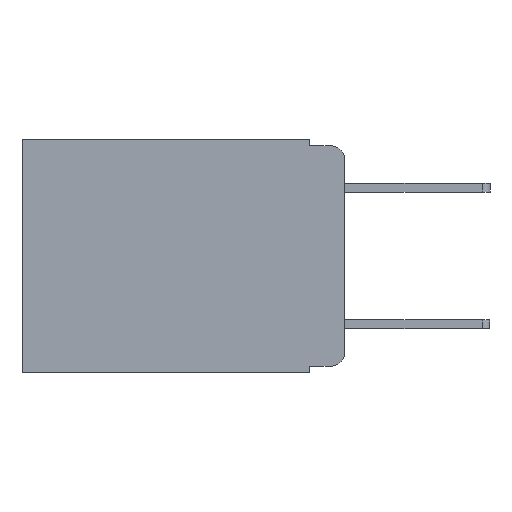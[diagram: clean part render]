
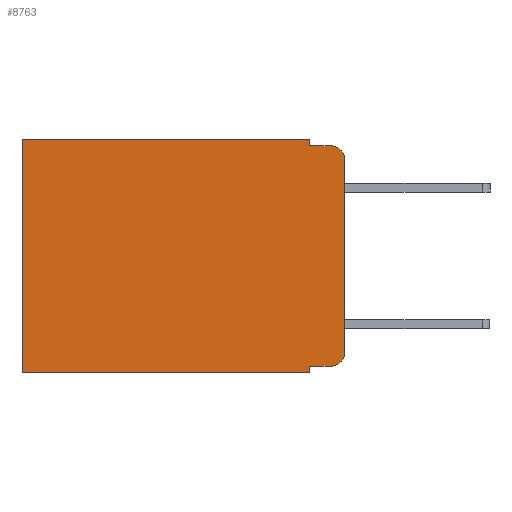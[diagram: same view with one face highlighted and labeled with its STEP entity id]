
A CAD part, left-side view. The second image highlights one B-rep face of the part: STEP entity #8763.
In plain terms, the highlighted planar face has unit normal (-1, 0, 0).
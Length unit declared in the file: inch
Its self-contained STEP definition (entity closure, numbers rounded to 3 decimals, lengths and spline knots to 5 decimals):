
#211 = VERTEX_POINT ( 'NONE', #2208 ) ;
#552 = DIRECTION ( 'NONE',  ( 0., 1., 0. ) ) ;
#572 = AXIS2_PLACEMENT_3D ( 'NONE', #5854, #4421, #10135 ) ;
#586 = CARTESIAN_POINT ( 'NONE',  ( 0.298, 0.051, -0.01 ) ) ;
#805 = VERTEX_POINT ( 'NONE', #586 ) ;
#829 = LINE ( 'NONE', #3305, #9333 ) ;
#880 = EDGE_CURVE ( 'NONE', #4049, #7673, #10518, .T. ) ;
#960 = CARTESIAN_POINT ( 'NONE',  ( 0.298, 0.051, 0. ) ) ;
#988 = EDGE_LOOP ( 'NONE', ( #2764, #4732, #3304, #2114, #5813, #4872, #7595, #1757, #4469, #1127 ) ) ;
#992 = EDGE_CURVE ( 'NONE', #5598, #4135, #9560, .T. ) ;
#1011 = EDGE_CURVE ( 'NONE', #8769, #5960, #829, .T. ) ;
#1127 = ORIENTED_EDGE ( 'NONE', *, *, #2802, .T. ) ;
#1315 = DIRECTION ( 'NONE',  ( 0., 0., -1. ) ) ;
#1406 = AXIS2_PLACEMENT_3D ( 'NONE', #4941, #5528, #5563 ) ;
#1739 = CARTESIAN_POINT ( 'NONE',  ( 0.298, 0.051, -0.343 ) ) ;
#1757 = ORIENTED_EDGE ( 'NONE', *, *, #4881, .F. ) ;
#1836 = VECTOR ( 'NONE', #6112, 39.37008 ) ;
#1850 = LINE ( 'NONE', #960, #3791 ) ;
#2114 = ORIENTED_EDGE ( 'NONE', *, *, #6151, .F. ) ;
#2208 = CARTESIAN_POINT ( 'NONE',  ( 0.298, 0.02, -0.01 ) ) ;
#2517 = CARTESIAN_POINT ( 'NONE',  ( 0.298, 0., -0.313 ) ) ;
#2719 = CARTESIAN_POINT ( 'NONE',  ( 0.298, 0.473, -0.343 ) ) ;
#2764 = ORIENTED_EDGE ( 'NONE', *, *, #992, .F. ) ;
#2770 = EDGE_CURVE ( 'NONE', #5598, #211, #2906, .T. ) ;
#2802 = EDGE_CURVE ( 'NONE', #5960, #4135, #6821, .T. ) ;
#2845 = LINE ( 'NONE', #7814, #9205 ) ;
#2900 = DIRECTION ( 'NONE',  ( 0., 1., 0. ) ) ;
#2906 = CIRCLE ( 'NONE', #9360, 0.02 ) ;
#3010 = VECTOR ( 'NONE', #2900, 39.37008 ) ;
#3304 = ORIENTED_EDGE ( 'NONE', *, *, #7318, .F. ) ;
#3305 = CARTESIAN_POINT ( 'NONE',  ( 0.298, 0.051, -0.333 ) ) ;
#3488 = CARTESIAN_POINT ( 'NONE',  ( 0.298, 0.051, -0.01 ) ) ;
#3596 = DIRECTION ( 'NONE',  ( 0., -1., 0. ) ) ;
#3791 = VECTOR ( 'NONE', #6749, 39.37008 ) ;
#4049 = VERTEX_POINT ( 'NONE', #9171 ) ;
#4135 = VERTEX_POINT ( 'NONE', #2517 ) ;
#4376 = VECTOR ( 'NONE', #552, 39.37008 ) ;
#4421 = DIRECTION ( 'NONE',  ( 1., 0., 0. ) ) ;
#4469 = ORIENTED_EDGE ( 'NONE', *, *, #1011, .T. ) ;
#4568 = CARTESIAN_POINT ( 'NONE',  ( 0.298, 0., 0. ) ) ;
#4732 = ORIENTED_EDGE ( 'NONE', *, *, #2770, .T. ) ;
#4779 = VECTOR ( 'NONE', #3596, 39.37008 ) ;
#4872 = ORIENTED_EDGE ( 'NONE', *, *, #880, .T. ) ;
#4881 = EDGE_CURVE ( 'NONE', #8769, #6019, #1850, .T. ) ;
#4941 = CARTESIAN_POINT ( 'NONE',  ( 0.298, 0.02, -0.313 ) ) ;
#5179 = PLANE ( 'NONE',  #572 ) ;
#5528 = DIRECTION ( 'NONE',  ( -1., 0., 0. ) ) ;
#5563 = DIRECTION ( 'NONE',  ( 0., 0., -1. ) ) ;
#5598 = VERTEX_POINT ( 'NONE', #7136 ) ;
#5813 = ORIENTED_EDGE ( 'NONE', *, *, #7146, .T. ) ;
#5854 = CARTESIAN_POINT ( 'NONE',  ( 0.298, 0., 0. ) ) ;
#5902 = CARTESIAN_POINT ( 'NONE',  ( 0.298, 0.02, -0.03 ) ) ;
#5960 = VERTEX_POINT ( 'NONE', #9818 ) ;
#6019 = VERTEX_POINT ( 'NONE', #1739 ) ;
#6112 = DIRECTION ( 'NONE',  ( 0., 0., -1. ) ) ;
#6151 = EDGE_CURVE ( 'NONE', #6370, #805, #2845, .T. ) ;
#6370 = VERTEX_POINT ( 'NONE', #7319 ) ;
#6503 = DIRECTION ( 'NONE',  ( 0., 0., -1. ) ) ;
#6531 = DIRECTION ( 'NONE',  ( -1., 0., 0. ) ) ;
#6749 = DIRECTION ( 'NONE',  ( 0., 0., -1. ) ) ;
#6821 = CIRCLE ( 'NONE', #1406, 0.02 ) ;
#6863 = LINE ( 'NONE', #9029, #4376 ) ;
#7136 = CARTESIAN_POINT ( 'NONE',  ( 0.298, 0., -0.03 ) ) ;
#7146 = EDGE_CURVE ( 'NONE', #6370, #4049, #6863, .T. ) ;
#7318 = EDGE_CURVE ( 'NONE', #805, #211, #9403, .T. ) ;
#7319 = CARTESIAN_POINT ( 'NONE',  ( 0.298, 0.051, 0. ) ) ;
#7443 = LINE ( 'NONE', #7925, #3010 ) ;
#7595 = ORIENTED_EDGE ( 'NONE', *, *, #9857, .F. ) ;
#7673 = VERTEX_POINT ( 'NONE', #2719 ) ;
#7814 = CARTESIAN_POINT ( 'NONE',  ( 0.298, 0.051, 0. ) ) ;
#7925 = CARTESIAN_POINT ( 'NONE',  ( 0.298, 0., -0.343 ) ) ;
#8554 = CARTESIAN_POINT ( 'NONE',  ( 0.298, 0.051, -0.333 ) ) ;
#8763 = ADVANCED_FACE ( 'NONE', ( #10216 ), #5179, .F. ) ;
#8769 = VERTEX_POINT ( 'NONE', #8554 ) ;
#8889 = DIRECTION ( 'NONE',  ( 0., 0., -1. ) ) ;
#9029 = CARTESIAN_POINT ( 'NONE',  ( 0.298, 0., 0. ) ) ;
#9171 = CARTESIAN_POINT ( 'NONE',  ( 0.298, 0.473, 0. ) ) ;
#9205 = VECTOR ( 'NONE', #8889, 39.37008 ) ;
#9333 = VECTOR ( 'NONE', #9604, 39.37008 ) ;
#9360 = AXIS2_PLACEMENT_3D ( 'NONE', #5902, #6531, #6503 ) ;
#9403 = LINE ( 'NONE', #3488, #4779 ) ;
#9560 = LINE ( 'NONE', #4568, #9819 ) ;
#9604 = DIRECTION ( 'NONE',  ( 0., -1., 0. ) ) ;
#9818 = CARTESIAN_POINT ( 'NONE',  ( 0.298, 0.02, -0.333 ) ) ;
#9819 = VECTOR ( 'NONE', #1315, 39.37008 ) ;
#9842 = CARTESIAN_POINT ( 'NONE',  ( 0.298, 0.473, 0. ) ) ;
#9857 = EDGE_CURVE ( 'NONE', #6019, #7673, #7443, .T. ) ;
#10135 = DIRECTION ( 'NONE',  ( 0., 0., -1. ) ) ;
#10216 = FACE_OUTER_BOUND ( 'NONE', #988, .T. ) ;
#10518 = LINE ( 'NONE', #9842, #1836 ) ;
